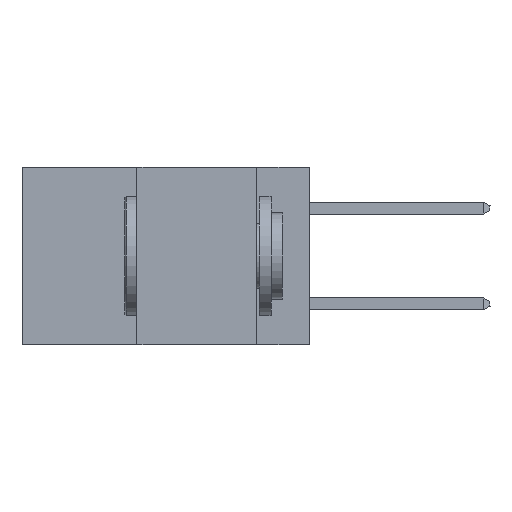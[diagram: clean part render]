
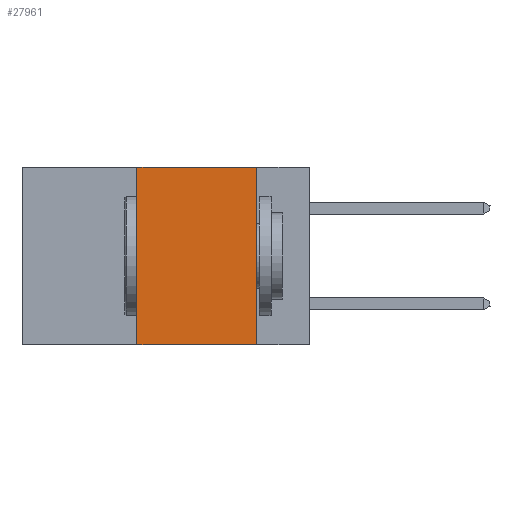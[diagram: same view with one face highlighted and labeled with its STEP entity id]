
A CAD part, left-side view. The second image highlights one B-rep face of the part: STEP entity #27961.
In plain terms, the highlighted planar face has unit normal (-1, 0, 0).
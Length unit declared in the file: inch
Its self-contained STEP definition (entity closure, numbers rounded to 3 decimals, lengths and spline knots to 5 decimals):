
#1288 = EDGE_LOOP ( 'NONE', ( #39493, #35729, #11282, #3498 ) ) ;
#2516 = VECTOR ( 'NONE', #19201, 39.37008 ) ;
#3091 = LINE ( 'NONE', #24979, #20407 ) ;
#3498 = ORIENTED_EDGE ( 'NONE', *, *, #39713, .T. ) ;
#3802 = CARTESIAN_POINT ( 'NONE',  ( 0., 0.36, -0.37 ) ) ;
#7765 = PLANE ( 'NONE',  #38105 ) ;
#8524 = LINE ( 'NONE', #18272, #31818 ) ;
#11282 = ORIENTED_EDGE ( 'NONE', *, *, #32361, .F. ) ;
#11917 = CARTESIAN_POINT ( 'NONE',  ( 0., 0.36, 0. ) ) ;
#14684 = EDGE_CURVE ( 'NONE', #39294, #27078, #33860, .T. ) ;
#16561 = DIRECTION ( 'NONE',  ( 0., 0., -1. ) ) ;
#17006 = FACE_OUTER_BOUND ( 'NONE', #1288, .T. ) ;
#18272 = CARTESIAN_POINT ( 'NONE',  ( 0., 0.6, 0. ) ) ;
#18538 = DIRECTION ( 'NONE',  ( 1., 0., 0. ) ) ;
#19201 = DIRECTION ( 'NONE',  ( 0., 0., 1. ) ) ;
#20407 = VECTOR ( 'NONE', #35570, 39.37008 ) ;
#20432 = CARTESIAN_POINT ( 'NONE',  ( 0., 0.11, 0. ) ) ;
#22156 = VERTEX_POINT ( 'NONE', #31702 ) ;
#24979 = CARTESIAN_POINT ( 'NONE',  ( 0., 0.6, -0.37 ) ) ;
#27078 = VERTEX_POINT ( 'NONE', #43780 ) ;
#27961 = ADVANCED_FACE ( 'NONE', ( #17006 ), #7765, .F. ) ;
#28100 = DIRECTION ( 'NONE',  ( 0., -1., 0. ) ) ;
#31702 = CARTESIAN_POINT ( 'NONE',  ( 0., 0.36, 0. ) ) ;
#31818 = VECTOR ( 'NONE', #28100, 39.37008 ) ;
#32361 = EDGE_CURVE ( 'NONE', #39483, #22156, #42613, .T. ) ;
#33860 = LINE ( 'NONE', #43946, #43591 ) ;
#35570 = DIRECTION ( 'NONE',  ( 0., -1., 0. ) ) ;
#35729 = ORIENTED_EDGE ( 'NONE', *, *, #38243, .F. ) ;
#35780 = CARTESIAN_POINT ( 'NONE',  ( 0., 0.6, 0. ) ) ;
#38105 = AXIS2_PLACEMENT_3D ( 'NONE', #35780, #18538, #42747 ) ;
#38243 = EDGE_CURVE ( 'NONE', #22156, #39294, #8524, .T. ) ;
#39294 = VERTEX_POINT ( 'NONE', #20432 ) ;
#39483 = VERTEX_POINT ( 'NONE', #3802 ) ;
#39493 = ORIENTED_EDGE ( 'NONE', *, *, #14684, .F. ) ;
#39713 = EDGE_CURVE ( 'NONE', #39483, #27078, #3091, .T. ) ;
#42613 = LINE ( 'NONE', #11917, #2516 ) ;
#42747 = DIRECTION ( 'NONE',  ( 0., 0., -1. ) ) ;
#43591 = VECTOR ( 'NONE', #16561, 39.37008 ) ;
#43780 = CARTESIAN_POINT ( 'NONE',  ( 0., 0.11, -0.37 ) ) ;
#43946 = CARTESIAN_POINT ( 'NONE',  ( 0., 0.11, 0. ) ) ;
